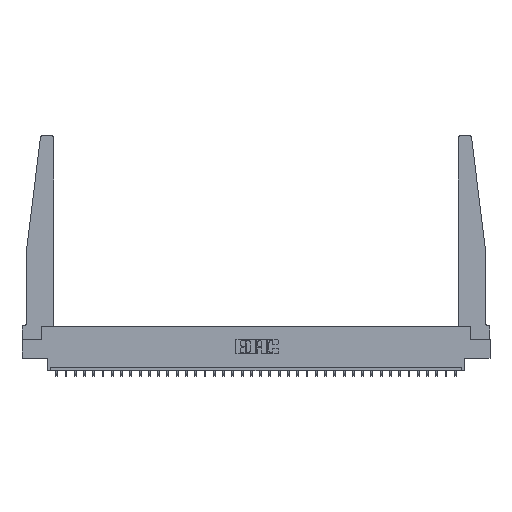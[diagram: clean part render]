
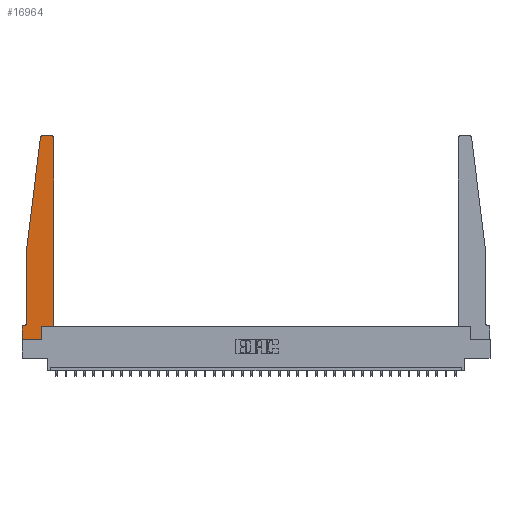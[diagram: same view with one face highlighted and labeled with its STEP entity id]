
A CAD part, top view. The second image highlights one B-rep face of the part: STEP entity #16964.
In plain terms, the highlighted planar face has unit normal (0, 0, 1).
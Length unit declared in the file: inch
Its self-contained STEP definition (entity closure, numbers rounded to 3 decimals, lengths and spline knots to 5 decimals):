
#106 = ORIENTED_EDGE ( 'NONE', *, *, #6142, .T. ) ;
#602 = AXIS2_PLACEMENT_3D ( 'NONE', #11129, #28282, #13610 ) ;
#727 = VERTEX_POINT ( 'NONE', #21659 ) ;
#794 = VECTOR ( 'NONE', #16321, 39.37008 ) ;
#1198 = CARTESIAN_POINT ( 'NONE',  ( 0.425, 0.18, 0.37 ) ) ;
#1679 = EDGE_CURVE ( 'NONE', #3298, #20881, #23360, .T. ) ;
#2052 = DIRECTION ( 'NONE',  ( 1., 0., 0. ) ) ;
#2661 = DIRECTION ( 'NONE',  ( 1., 0., 0. ) ) ;
#3148 = LINE ( 'NONE', #30110, #9041 ) ;
#3186 = CIRCLE ( 'NONE', #602, 0.05 ) ;
#3298 = VERTEX_POINT ( 'NONE', #12682 ) ;
#3377 = ORIENTED_EDGE ( 'NONE', *, *, #19495, .T. ) ;
#3673 = ORIENTED_EDGE ( 'NONE', *, *, #13565, .T. ) ;
#4091 = CIRCLE ( 'NONE', #15175, 0.03 ) ;
#4139 = CARTESIAN_POINT ( 'NONE',  ( 0., 0.1875, 0.37 ) ) ;
#4253 = DIRECTION ( 'NONE',  ( 0., 0., 1. ) ) ;
#4765 = CARTESIAN_POINT ( 'NONE',  ( 0.24675, 2.72367, 0.37 ) ) ;
#5218 = DIRECTION ( 'NONE',  ( 0., 1., 0. ) ) ;
#5268 = CARTESIAN_POINT ( 'NONE',  ( 0.2605, 0., 0.37 ) ) ;
#5915 = LINE ( 'NONE', #31014, #794 ) ;
#6142 = EDGE_CURVE ( 'NONE', #25962, #3298, #3186, .T. ) ;
#6478 = LINE ( 'NONE', #24226, #26116 ) ;
#6627 = DIRECTION ( 'NONE',  ( 0., 1., 0. ) ) ;
#6669 = LINE ( 'NONE', #19955, #19744 ) ;
#7164 = EDGE_CURVE ( 'NONE', #22873, #727, #6669, .T. ) ;
#7273 = LINE ( 'NONE', #15061, #19570 ) ;
#8340 = DIRECTION ( 'NONE',  ( -1., 0., 0. ) ) ;
#8615 = ORIENTED_EDGE ( 'NONE', *, *, #1679, .T. ) ;
#8776 = CARTESIAN_POINT ( 'NONE',  ( 0.2605, 0.18, 0.37 ) ) ;
#8858 = ORIENTED_EDGE ( 'NONE', *, *, #17073, .T. ) ;
#8897 = ORIENTED_EDGE ( 'NONE', *, *, #14429, .T. ) ;
#9041 = VECTOR ( 'NONE', #17761, 39.37008 ) ;
#9144 = CARTESIAN_POINT ( 'NONE',  ( 0.2605, 0.18, 0.37 ) ) ;
#9279 = EDGE_CURVE ( 'NONE', #12038, #17736, #31984, .T. ) ;
#10218 = AXIS2_PLACEMENT_3D ( 'NONE', #4139, #4253, #21506 ) ;
#10486 = AXIS2_PLACEMENT_3D ( 'NONE', #26511, #11832, #28964 ) ;
#10533 = EDGE_CURVE ( 'NONE', #14217, #21397, #7273, .T. ) ;
#11129 = CARTESIAN_POINT ( 'NONE',  ( 0.015, 0.2375, 0.37 ) ) ;
#11832 = DIRECTION ( 'NONE',  ( 0., 0., 1. ) ) ;
#12038 = VERTEX_POINT ( 'NONE', #15398 ) ;
#12682 = CARTESIAN_POINT ( 'NONE',  ( 0.015, 0.1875, 0.37 ) ) ;
#13565 = EDGE_CURVE ( 'NONE', #21397, #16233, #14128, .T. ) ;
#13610 = DIRECTION ( 'NONE',  ( -1., 0., 0. ) ) ;
#14128 = LINE ( 'NONE', #9144, #19829 ) ;
#14136 = DIRECTION ( 'NONE',  ( -1., 0., 0. ) ) ;
#14217 = VERTEX_POINT ( 'NONE', #24377 ) ;
#14429 = EDGE_CURVE ( 'NONE', #20881, #14217, #3148, .T. ) ;
#14562 = CARTESIAN_POINT ( 'NONE',  ( 0.395, 2.72, 0.37 ) ) ;
#15061 = CARTESIAN_POINT ( 'NONE',  ( 0., 0., 0.37 ) ) ;
#15175 = AXIS2_PLACEMENT_3D ( 'NONE', #14562, #31713, #16995 ) ;
#15398 = CARTESIAN_POINT ( 'NONE',  ( 0.27653, 2.75, 0.37 ) ) ;
#16233 = VERTEX_POINT ( 'NONE', #8776 ) ;
#16321 = DIRECTION ( 'NONE',  ( 0., -1., 0. ) ) ;
#16574 = PLANE ( 'NONE',  #10218 ) ;
#16964 = ADVANCED_FACE ( 'NONE', ( #26204 ), #16574, .T. ) ;
#16995 = DIRECTION ( 'NONE',  ( 1., 0., 0. ) ) ;
#17073 = EDGE_CURVE ( 'NONE', #727, #17584, #4091, .T. ) ;
#17240 = ORIENTED_EDGE ( 'NONE', *, *, #17854, .T. ) ;
#17584 = VERTEX_POINT ( 'NONE', #18989 ) ;
#17736 = VERTEX_POINT ( 'NONE', #4765 ) ;
#17761 = DIRECTION ( 'NONE',  ( 0., -1., 0. ) ) ;
#17854 = EDGE_CURVE ( 'NONE', #17736, #20462, #31004, .T. ) ;
#18684 = ORIENTED_EDGE ( 'NONE', *, *, #10533, .T. ) ;
#18989 = CARTESIAN_POINT ( 'NONE',  ( 0.395, 2.75, 0.37 ) ) ;
#19495 = EDGE_CURVE ( 'NONE', #17584, #12038, #29398, .T. ) ;
#19570 = VECTOR ( 'NONE', #2661, 39.37008 ) ;
#19744 = VECTOR ( 'NONE', #5218, 39.37008 ) ;
#19829 = VECTOR ( 'NONE', #6627, 39.37008 ) ;
#19931 = DIRECTION ( 'NONE',  ( -0.122, -0.992, 0. ) ) ;
#19955 = CARTESIAN_POINT ( 'NONE',  ( 0.425, 0.18, 0.37 ) ) ;
#20462 = VERTEX_POINT ( 'NONE', #22532 ) ;
#20755 = ORIENTED_EDGE ( 'NONE', *, *, #7164, .T. ) ;
#20881 = VERTEX_POINT ( 'NONE', #26362 ) ;
#21397 = VERTEX_POINT ( 'NONE', #5268 ) ;
#21506 = DIRECTION ( 'NONE',  ( 1., 0., 0. ) ) ;
#21659 = CARTESIAN_POINT ( 'NONE',  ( 0.425, 2.72, 0.37 ) ) ;
#22532 = CARTESIAN_POINT ( 'NONE',  ( 0.065, 1.25, 0.37 ) ) ;
#22873 = VERTEX_POINT ( 'NONE', #1198 ) ;
#22913 = VECTOR ( 'NONE', #14136, 39.37008 ) ;
#23360 = LINE ( 'NONE', #27977, #29080 ) ;
#23640 = CARTESIAN_POINT ( 'NONE',  ( 0.065, 0.2375, 0.37 ) ) ;
#23686 = EDGE_CURVE ( 'NONE', #16233, #22873, #6478, .T. ) ;
#24226 = CARTESIAN_POINT ( 'NONE',  ( 0.425, 0.18, 0.37 ) ) ;
#24377 = CARTESIAN_POINT ( 'NONE',  ( 0., 0., 0.37 ) ) ;
#24509 = VECTOR ( 'NONE', #19931, 39.37008 ) ;
#25954 = EDGE_CURVE ( 'NONE', #20462, #25962, #5915, .T. ) ;
#25962 = VERTEX_POINT ( 'NONE', #23640 ) ;
#26116 = VECTOR ( 'NONE', #2052, 39.37008 ) ;
#26204 = FACE_OUTER_BOUND ( 'NONE', #28098, .T. ) ;
#26345 = ORIENTED_EDGE ( 'NONE', *, *, #25954, .T. ) ;
#26362 = CARTESIAN_POINT ( 'NONE',  ( 0., 0.1875, 0.37 ) ) ;
#26511 = CARTESIAN_POINT ( 'NONE',  ( 0.27653, 2.72, 0.37 ) ) ;
#27977 = CARTESIAN_POINT ( 'NONE',  ( 0.065, 0.1875, 0.37 ) ) ;
#28098 = EDGE_LOOP ( 'NONE', ( #3377, #31657, #17240, #26345, #106, #8615, #8897, #18684, #3673, #29850, #20755, #8858 ) ) ;
#28282 = DIRECTION ( 'NONE',  ( 0., 0., -1. ) ) ;
#28964 = DIRECTION ( 'NONE',  ( 1., 0., 0. ) ) ;
#29080 = VECTOR ( 'NONE', #8340, 39.37008 ) ;
#29398 = LINE ( 'NONE', #31281, #22913 ) ;
#29809 = CARTESIAN_POINT ( 'NONE',  ( 0.065, 1.25, 0.37 ) ) ;
#29850 = ORIENTED_EDGE ( 'NONE', *, *, #23686, .T. ) ;
#30110 = CARTESIAN_POINT ( 'NONE',  ( 0., 0., 0.37 ) ) ;
#31004 = LINE ( 'NONE', #29809, #24509 ) ;
#31014 = CARTESIAN_POINT ( 'NONE',  ( 0.065, 1.25, 0.37 ) ) ;
#31281 = CARTESIAN_POINT ( 'NONE',  ( 0.25, 2.75, 0.37 ) ) ;
#31657 = ORIENTED_EDGE ( 'NONE', *, *, #9279, .T. ) ;
#31713 = DIRECTION ( 'NONE',  ( 0., 0., 1. ) ) ;
#31984 = CIRCLE ( 'NONE', #10486, 0.03 ) ;
